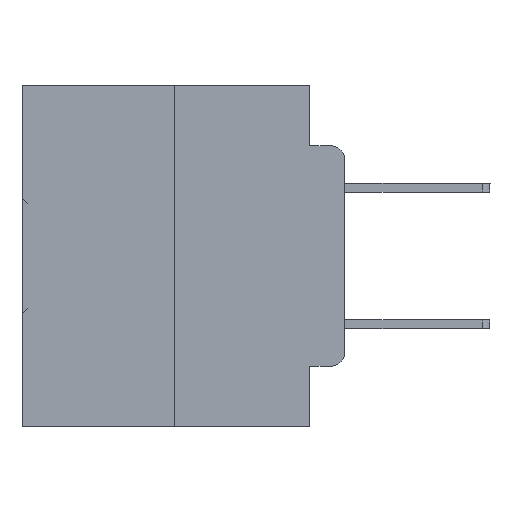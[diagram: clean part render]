
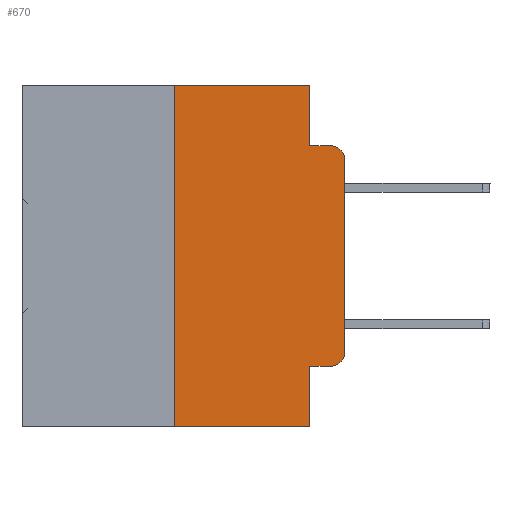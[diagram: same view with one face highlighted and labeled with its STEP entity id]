
A CAD part, left-side view. The second image highlights one B-rep face of the part: STEP entity #670.
In plain terms, the highlighted planar face has unit normal (-1, 0, 0).
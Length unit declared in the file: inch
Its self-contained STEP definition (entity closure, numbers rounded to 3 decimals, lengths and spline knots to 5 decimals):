
#670 = ADVANCED_FACE ( 'NONE', ( #16292 ), #14319, .F. ) ;
#779 = VECTOR ( 'NONE', #25604, 39.37008 ) ;
#959 = CARTESIAN_POINT ( 'NONE',  ( 0., 0.051, -0.4115 ) ) ;
#971 = CARTESIAN_POINT ( 'NONE',  ( 0., 0.02, -0.0885 ) ) ;
#1082 = ORIENTED_EDGE ( 'NONE', *, *, #15611, .T. ) ;
#2075 = EDGE_CURVE ( 'NONE', #11682, #15037, #9616, .T. ) ;
#2239 = VERTEX_POINT ( 'NONE', #13473 ) ;
#2300 = ORIENTED_EDGE ( 'NONE', *, *, #31478, .F. ) ;
#2557 = ORIENTED_EDGE ( 'NONE', *, *, #34652, .F. ) ;
#3449 = VERTEX_POINT ( 'NONE', #10866 ) ;
#3824 = EDGE_CURVE ( 'NONE', #20343, #11682, #12657, .T. ) ;
#4003 = EDGE_CURVE ( 'NONE', #5915, #3449, #8227, .T. ) ;
#4101 = CIRCLE ( 'NONE', #18079, 0.02 ) ;
#5584 = ORIENTED_EDGE ( 'NONE', *, *, #12076, .F. ) ;
#5915 = VERTEX_POINT ( 'NONE', #959 ) ;
#6232 = EDGE_CURVE ( 'NONE', #14638, #3449, #26993, .T. ) ;
#6554 = VECTOR ( 'NONE', #14242, 39.37008 ) ;
#6781 = CARTESIAN_POINT ( 'NONE',  ( 0., 0., 0. ) ) ;
#6883 = CARTESIAN_POINT ( 'NONE',  ( 0., 0.25, 0. ) ) ;
#7532 = CARTESIAN_POINT ( 'NONE',  ( 0., 0.02, -0.1085 ) ) ;
#8227 = LINE ( 'NONE', #22808, #779 ) ;
#8656 = ORIENTED_EDGE ( 'NONE', *, *, #3824, .T. ) ;
#9020 = EDGE_LOOP ( 'NONE', ( #8656, #14026, #2300, #2557, #18378, #5584, #19024, #25088, #20382, #1082 ) ) ;
#9412 = DIRECTION ( 'NONE',  ( 1., 0., 0. ) ) ;
#9616 = CIRCLE ( 'NONE', #11949, 0.02 ) ;
#9907 = DIRECTION ( 'NONE',  ( 0., -1., 0. ) ) ;
#10382 = VERTEX_POINT ( 'NONE', #6883 ) ;
#10443 = VERTEX_POINT ( 'NONE', #35128 ) ;
#10458 = VECTOR ( 'NONE', #17252, 39.37008 ) ;
#10498 = DIRECTION ( 'NONE',  ( 0., 0., -1. ) ) ;
#10866 = CARTESIAN_POINT ( 'NONE',  ( 0., 0.051, -0.5 ) ) ;
#10996 = DIRECTION ( 'NONE',  ( 0., -1., 0. ) ) ;
#11682 = VERTEX_POINT ( 'NONE', #18332 ) ;
#11719 = VECTOR ( 'NONE', #23303, 39.37008 ) ;
#11755 = DIRECTION ( 'NONE',  ( 0., 0., -1. ) ) ;
#11949 = AXIS2_PLACEMENT_3D ( 'NONE', #7532, #24406, #10498 ) ;
#12076 = EDGE_CURVE ( 'NONE', #14638, #10382, #32725, .T. ) ;
#12460 = DIRECTION ( 'NONE',  ( 0., 0., 1. ) ) ;
#12612 = CARTESIAN_POINT ( 'NONE',  ( 0., 0.051, -0.0885 ) ) ;
#12657 = LINE ( 'NONE', #6781, #19194 ) ;
#13473 = CARTESIAN_POINT ( 'NONE',  ( 0., 0.051, 0. ) ) ;
#14026 = ORIENTED_EDGE ( 'NONE', *, *, #2075, .T. ) ;
#14242 = DIRECTION ( 'NONE',  ( 0., -1., 0. ) ) ;
#14319 = PLANE ( 'NONE',  #34103 ) ;
#14638 = VERTEX_POINT ( 'NONE', #22954 ) ;
#14909 = DIRECTION ( 'NONE',  ( 0., 0., -1. ) ) ;
#15037 = VERTEX_POINT ( 'NONE', #971 ) ;
#15611 = EDGE_CURVE ( 'NONE', #10443, #20343, #4101, .T. ) ;
#16292 = FACE_OUTER_BOUND ( 'NONE', #9020, .T. ) ;
#17252 = DIRECTION ( 'NONE',  ( 0., 0., 1. ) ) ;
#17732 = DIRECTION ( 'NONE',  ( 0., -1., 0. ) ) ;
#17810 = CARTESIAN_POINT ( 'NONE',  ( 0., 0.051, 0. ) ) ;
#18079 = AXIS2_PLACEMENT_3D ( 'NONE', #31947, #23557, #14909 ) ;
#18332 = CARTESIAN_POINT ( 'NONE',  ( 0., 0., -0.1085 ) ) ;
#18378 = ORIENTED_EDGE ( 'NONE', *, *, #18804, .F. ) ;
#18804 = EDGE_CURVE ( 'NONE', #10382, #2239, #36115, .T. ) ;
#19024 = ORIENTED_EDGE ( 'NONE', *, *, #6232, .T. ) ;
#19194 = VECTOR ( 'NONE', #12460, 39.37008 ) ;
#19316 = VECTOR ( 'NONE', #9907, 39.37008 ) ;
#19471 = CARTESIAN_POINT ( 'NONE',  ( 0., 0., -0.3915 ) ) ;
#20343 = VERTEX_POINT ( 'NONE', #19471 ) ;
#20382 = ORIENTED_EDGE ( 'NONE', *, *, #27246, .T. ) ;
#21987 = CARTESIAN_POINT ( 'NONE',  ( 0., 0.473, -0.5 ) ) ;
#22804 = CARTESIAN_POINT ( 'NONE',  ( 0., 0.051, -0.0885 ) ) ;
#22808 = CARTESIAN_POINT ( 'NONE',  ( 0., 0.051, 0. ) ) ;
#22954 = CARTESIAN_POINT ( 'NONE',  ( 0., 0.25, -0.5 ) ) ;
#23303 = DIRECTION ( 'NONE',  ( 0., 0., -1. ) ) ;
#23557 = DIRECTION ( 'NONE',  ( -1., 0., 0. ) ) ;
#24406 = DIRECTION ( 'NONE',  ( -1., 0., 0. ) ) ;
#25088 = ORIENTED_EDGE ( 'NONE', *, *, #4003, .F. ) ;
#25604 = DIRECTION ( 'NONE',  ( 0., 0., -1. ) ) ;
#26993 = LINE ( 'NONE', #21987, #33080 ) ;
#27246 = EDGE_CURVE ( 'NONE', #5915, #10443, #31036, .T. ) ;
#27622 = LINE ( 'NONE', #12612, #19316 ) ;
#28681 = VECTOR ( 'NONE', #17732, 39.37008 ) ;
#30049 = LINE ( 'NONE', #17810, #11719 ) ;
#30680 = VERTEX_POINT ( 'NONE', #22804 ) ;
#31036 = LINE ( 'NONE', #33495, #6554 ) ;
#31478 = EDGE_CURVE ( 'NONE', #30680, #15037, #27622, .T. ) ;
#31614 = CARTESIAN_POINT ( 'NONE',  ( 0., 0.473, 0. ) ) ;
#31947 = CARTESIAN_POINT ( 'NONE',  ( 0., 0.02, -0.3915 ) ) ;
#32725 = LINE ( 'NONE', #34093, #10458 ) ;
#33080 = VECTOR ( 'NONE', #10996, 39.37008 ) ;
#33495 = CARTESIAN_POINT ( 'NONE',  ( 0., 0.051, -0.4115 ) ) ;
#33826 = CARTESIAN_POINT ( 'NONE',  ( 0., 0.473, 0. ) ) ;
#34093 = CARTESIAN_POINT ( 'NONE',  ( 0., 0.25, 0. ) ) ;
#34103 = AXIS2_PLACEMENT_3D ( 'NONE', #33826, #9412, #11755 ) ;
#34652 = EDGE_CURVE ( 'NONE', #2239, #30680, #30049, .T. ) ;
#35128 = CARTESIAN_POINT ( 'NONE',  ( 0., 0.02, -0.4115 ) ) ;
#36115 = LINE ( 'NONE', #31614, #28681 ) ;
